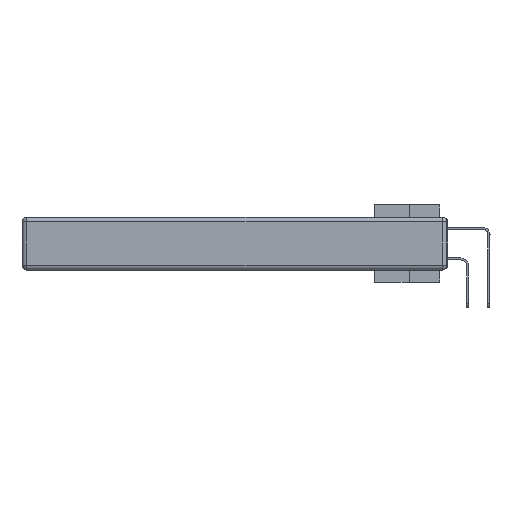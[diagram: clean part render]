
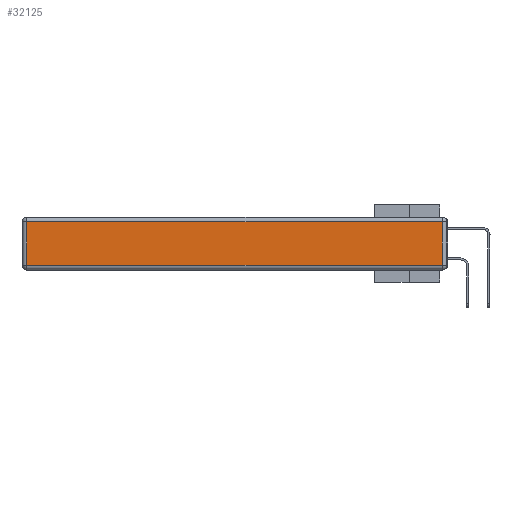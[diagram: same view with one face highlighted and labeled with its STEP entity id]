
A CAD part, left-side view. The second image highlights one B-rep face of the part: STEP entity #32125.
In plain terms, the highlighted planar face has unit normal (-1, 0, 0).
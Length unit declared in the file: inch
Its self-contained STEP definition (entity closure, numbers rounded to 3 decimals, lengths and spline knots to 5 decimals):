
#351 = CARTESIAN_POINT ( 'NONE',  ( 0., 0.03, -0.313 ) ) ;
#873 = CARTESIAN_POINT ( 'NONE',  ( 0., 0.03, -0.343 ) ) ;
#1565 = EDGE_CURVE ( 'NONE', #5121, #3101, #8645, .T. ) ;
#2137 = VECTOR ( 'NONE', #6347, 39.37008 ) ;
#2364 = PLANE ( 'NONE',  #11247 ) ;
#3101 = VERTEX_POINT ( 'NONE', #351 ) ;
#3162 = EDGE_CURVE ( 'NONE', #32473, #5121, #27621, .T. ) ;
#3648 = FACE_OUTER_BOUND ( 'NONE', #7907, .T. ) ;
#4452 = VECTOR ( 'NONE', #17987, 39.37008 ) ;
#5121 = VERTEX_POINT ( 'NONE', #28143 ) ;
#6347 = DIRECTION ( 'NONE',  ( 0., 1., 0. ) ) ;
#6510 = CARTESIAN_POINT ( 'NONE',  ( 0., 0.03, -0.03 ) ) ;
#7742 = VECTOR ( 'NONE', #12034, 39.37008 ) ;
#7743 = ORIENTED_EDGE ( 'NONE', *, *, #30498, .T. ) ;
#7907 = EDGE_LOOP ( 'NONE', ( #26298, #7743, #24528, #19577 ) ) ;
#8645 = LINE ( 'NONE', #35745, #7742 ) ;
#8745 = VERTEX_POINT ( 'NONE', #6510 ) ;
#9630 = LINE ( 'NONE', #873, #23280 ) ;
#11247 = AXIS2_PLACEMENT_3D ( 'NONE', #28558, #31763, #33574 ) ;
#12034 = DIRECTION ( 'NONE',  ( 0., -1., 0. ) ) ;
#17119 = LINE ( 'NONE', #18037, #2137 ) ;
#17987 = DIRECTION ( 'NONE',  ( 0., 0., -1. ) ) ;
#18037 = CARTESIAN_POINT ( 'NONE',  ( 0., 2.75, -0.03 ) ) ;
#19577 = ORIENTED_EDGE ( 'NONE', *, *, #3162, .T. ) ;
#22400 = EDGE_CURVE ( 'NONE', #8745, #32473, #17119, .T. ) ;
#23280 = VECTOR ( 'NONE', #29973, 39.37008 ) ;
#24528 = ORIENTED_EDGE ( 'NONE', *, *, #22400, .T. ) ;
#26298 = ORIENTED_EDGE ( 'NONE', *, *, #1565, .T. ) ;
#27621 = LINE ( 'NONE', #29679, #4452 ) ;
#28143 = CARTESIAN_POINT ( 'NONE',  ( 0., 2.72, -0.313 ) ) ;
#28558 = CARTESIAN_POINT ( 'NONE',  ( 0., 0., -0.343 ) ) ;
#29679 = CARTESIAN_POINT ( 'NONE',  ( 0., 2.72, -0.343 ) ) ;
#29973 = DIRECTION ( 'NONE',  ( 0., 0., 1. ) ) ;
#30498 = EDGE_CURVE ( 'NONE', #3101, #8745, #9630, .T. ) ;
#31763 = DIRECTION ( 'NONE',  ( -1., 0., 0. ) ) ;
#32125 = ADVANCED_FACE ( 'NONE', ( #3648 ), #2364, .T. ) ;
#32473 = VERTEX_POINT ( 'NONE', #36217 ) ;
#33574 = DIRECTION ( 'NONE',  ( 0., 0., 1. ) ) ;
#35745 = CARTESIAN_POINT ( 'NONE',  ( 0., 0., -0.313 ) ) ;
#36217 = CARTESIAN_POINT ( 'NONE',  ( 0., 2.72, -0.03 ) ) ;
